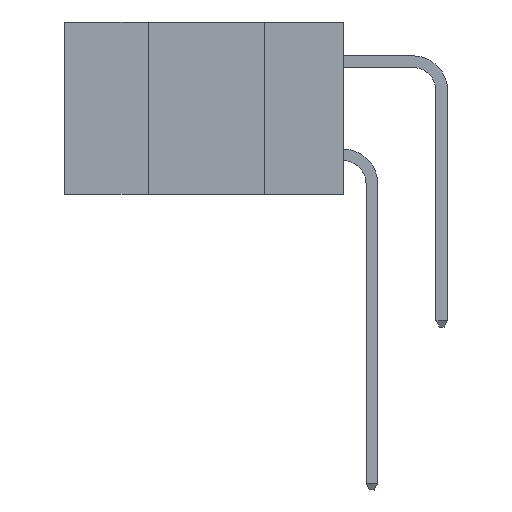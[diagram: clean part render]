
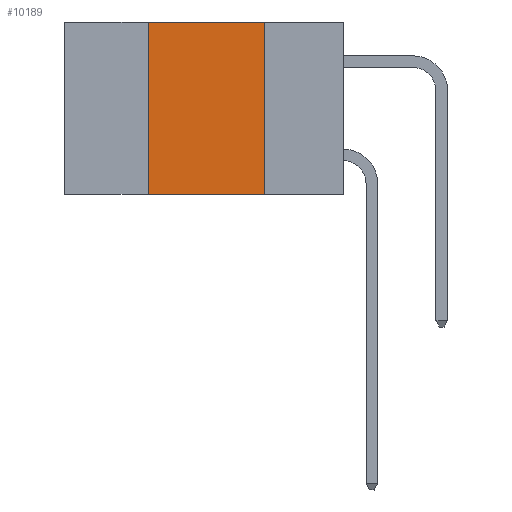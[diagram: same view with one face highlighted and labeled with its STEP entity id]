
A CAD part, left-side view. The second image highlights one B-rep face of the part: STEP entity #10189.
In plain terms, the highlighted planar face has unit normal (-1, 0, 0).
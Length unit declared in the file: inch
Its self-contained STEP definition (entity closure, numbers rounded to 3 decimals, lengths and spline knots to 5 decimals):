
#1259 = VERTEX_POINT ( 'NONE', #2129 ) ;
#1348 = PLANE ( 'NONE',  #4239 ) ;
#1800 = EDGE_LOOP ( 'NONE', ( #14961, #6511, #3048, #9342 ) ) ;
#1851 = DIRECTION ( 'NONE',  ( 0., 0., -1. ) ) ;
#1906 = CARTESIAN_POINT ( 'NONE',  ( 0., 0.6, 0. ) ) ;
#2129 = CARTESIAN_POINT ( 'NONE',  ( 0., 0.42, 0. ) ) ;
#2490 = DIRECTION ( 'NONE',  ( 0., 0., -1. ) ) ;
#2767 = CARTESIAN_POINT ( 'NONE',  ( 0., 0.17, -0.37 ) ) ;
#2849 = VECTOR ( 'NONE', #6806, 39.37008 ) ;
#3048 = ORIENTED_EDGE ( 'NONE', *, *, #6452, .F. ) ;
#3140 = VECTOR ( 'NONE', #1851, 39.37008 ) ;
#3507 = LINE ( 'NONE', #11276, #3140 ) ;
#3543 = DIRECTION ( 'NONE',  ( 0., 0., 1. ) ) ;
#4239 = AXIS2_PLACEMENT_3D ( 'NONE', #11765, #9501, #2490 ) ;
#5373 = DIRECTION ( 'NONE',  ( 0., -1., 0. ) ) ;
#5633 = CARTESIAN_POINT ( 'NONE',  ( 0., 0.6, -0.37 ) ) ;
#6452 = EDGE_CURVE ( 'NONE', #10167, #1259, #13380, .T. ) ;
#6511 = ORIENTED_EDGE ( 'NONE', *, *, #9872, .F. ) ;
#6706 = VERTEX_POINT ( 'NONE', #2767 ) ;
#6806 = DIRECTION ( 'NONE',  ( 0., -1., 0. ) ) ;
#7372 = VERTEX_POINT ( 'NONE', #13285 ) ;
#8113 = EDGE_CURVE ( 'NONE', #7372, #6706, #3507, .T. ) ;
#9073 = LINE ( 'NONE', #5633, #2849 ) ;
#9342 = ORIENTED_EDGE ( 'NONE', *, *, #14023, .T. ) ;
#9501 = DIRECTION ( 'NONE',  ( 1., 0., 0. ) ) ;
#9557 = LINE ( 'NONE', #1906, #12257 ) ;
#9872 = EDGE_CURVE ( 'NONE', #1259, #7372, #9557, .T. ) ;
#10167 = VERTEX_POINT ( 'NONE', #10616 ) ;
#10189 = ADVANCED_FACE ( 'NONE', ( #11354 ), #1348, .F. ) ;
#10324 = VECTOR ( 'NONE', #3543, 39.37008 ) ;
#10616 = CARTESIAN_POINT ( 'NONE',  ( 0., 0.42, -0.37 ) ) ;
#11276 = CARTESIAN_POINT ( 'NONE',  ( 0., 0.17, 0. ) ) ;
#11354 = FACE_OUTER_BOUND ( 'NONE', #1800, .T. ) ;
#11765 = CARTESIAN_POINT ( 'NONE',  ( 0., 0.6, 0. ) ) ;
#12257 = VECTOR ( 'NONE', #5373, 39.37008 ) ;
#12854 = CARTESIAN_POINT ( 'NONE',  ( 0., 0.42, 0. ) ) ;
#13285 = CARTESIAN_POINT ( 'NONE',  ( 0., 0.17, 0. ) ) ;
#13380 = LINE ( 'NONE', #12854, #10324 ) ;
#14023 = EDGE_CURVE ( 'NONE', #10167, #6706, #9073, .T. ) ;
#14961 = ORIENTED_EDGE ( 'NONE', *, *, #8113, .F. ) ;
